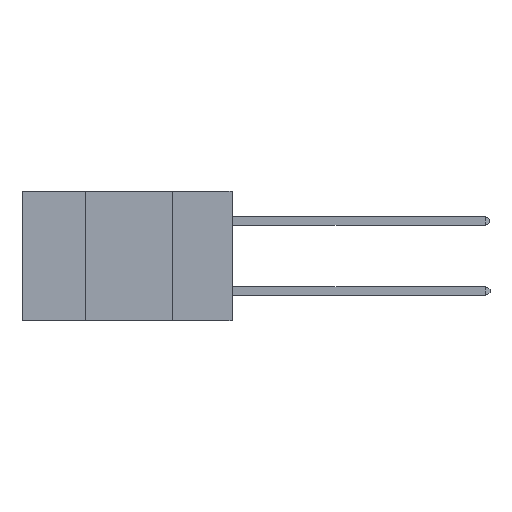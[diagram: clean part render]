
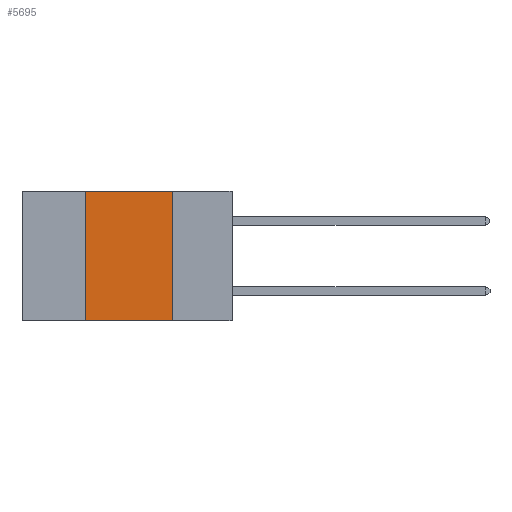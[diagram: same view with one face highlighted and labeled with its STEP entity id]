
A CAD part, left-side view. The second image highlights one B-rep face of the part: STEP entity #5695.
In plain terms, the highlighted planar face has unit normal (-1, 0, 0).
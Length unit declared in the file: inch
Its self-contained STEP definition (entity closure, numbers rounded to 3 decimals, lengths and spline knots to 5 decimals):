
#121 = EDGE_CURVE ( 'NONE', #169, #6486, #18727, .T. ) ;
#169 = VERTEX_POINT ( 'NONE', #18043 ) ;
#624 = LINE ( 'NONE', #840, #21607 ) ;
#840 = CARTESIAN_POINT ( 'NONE',  ( 0., 0.42, 0. ) ) ;
#2241 = VECTOR ( 'NONE', #17099, 39.37008 ) ;
#2352 = ORIENTED_EDGE ( 'NONE', *, *, #7388, .F. ) ;
#3039 = EDGE_LOOP ( 'NONE', ( #7017, #3951, #2352, #23675 ) ) ;
#3174 = CARTESIAN_POINT ( 'NONE',  ( 0., 0.42, 0. ) ) ;
#3795 = EDGE_CURVE ( 'NONE', #11135, #6486, #12896, .T. ) ;
#3951 = ORIENTED_EDGE ( 'NONE', *, *, #5454, .F. ) ;
#4577 = DIRECTION ( 'NONE',  ( 0., 0., 1. ) ) ;
#5454 = EDGE_CURVE ( 'NONE', #6936, #169, #17219, .T. ) ;
#5622 = DIRECTION ( 'NONE',  ( 0., 0., -1. ) ) ;
#5695 = ADVANCED_FACE ( 'NONE', ( #11680 ), #18491, .F. ) ;
#6486 = VERTEX_POINT ( 'NONE', #16617 ) ;
#6544 = DIRECTION ( 'NONE',  ( 0., 0., -1. ) ) ;
#6936 = VERTEX_POINT ( 'NONE', #3174 ) ;
#7017 = ORIENTED_EDGE ( 'NONE', *, *, #121, .F. ) ;
#7388 = EDGE_CURVE ( 'NONE', #11135, #6936, #624, .T. ) ;
#7935 = CARTESIAN_POINT ( 'NONE',  ( 0., 0.6, -0.37 ) ) ;
#8026 = DIRECTION ( 'NONE',  ( 0., -1., 0. ) ) ;
#11108 = CARTESIAN_POINT ( 'NONE',  ( 0., 0.6, 0. ) ) ;
#11135 = VERTEX_POINT ( 'NONE', #17500 ) ;
#11680 = FACE_OUTER_BOUND ( 'NONE', #3039, .T. ) ;
#11967 = VECTOR ( 'NONE', #8026, 39.37008 ) ;
#12896 = LINE ( 'NONE', #7935, #2241 ) ;
#14069 = CARTESIAN_POINT ( 'NONE',  ( 0., 0.17, 0. ) ) ;
#16617 = CARTESIAN_POINT ( 'NONE',  ( 0., 0.17, -0.37 ) ) ;
#16731 = DIRECTION ( 'NONE',  ( 1., 0., 0. ) ) ;
#17099 = DIRECTION ( 'NONE',  ( 0., -1., 0. ) ) ;
#17219 = LINE ( 'NONE', #20905, #11967 ) ;
#17500 = CARTESIAN_POINT ( 'NONE',  ( 0., 0.42, -0.37 ) ) ;
#18043 = CARTESIAN_POINT ( 'NONE',  ( 0., 0.17, 0. ) ) ;
#18491 = PLANE ( 'NONE',  #23610 ) ;
#18727 = LINE ( 'NONE', #14069, #19575 ) ;
#19575 = VECTOR ( 'NONE', #6544, 39.37008 ) ;
#20905 = CARTESIAN_POINT ( 'NONE',  ( 0., 0.6, 0. ) ) ;
#21607 = VECTOR ( 'NONE', #4577, 39.37008 ) ;
#23610 = AXIS2_PLACEMENT_3D ( 'NONE', #11108, #16731, #5622 ) ;
#23675 = ORIENTED_EDGE ( 'NONE', *, *, #3795, .T. ) ;
